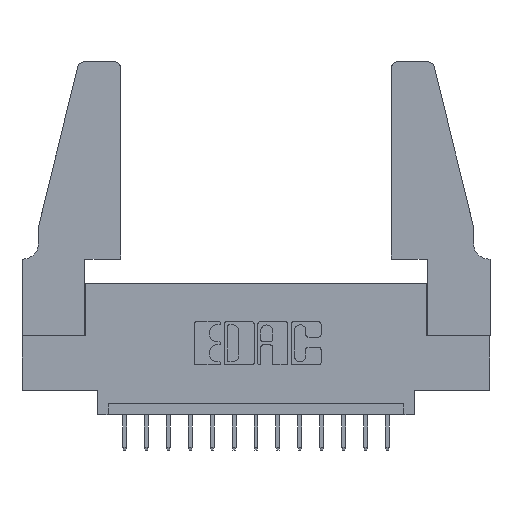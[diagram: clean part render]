
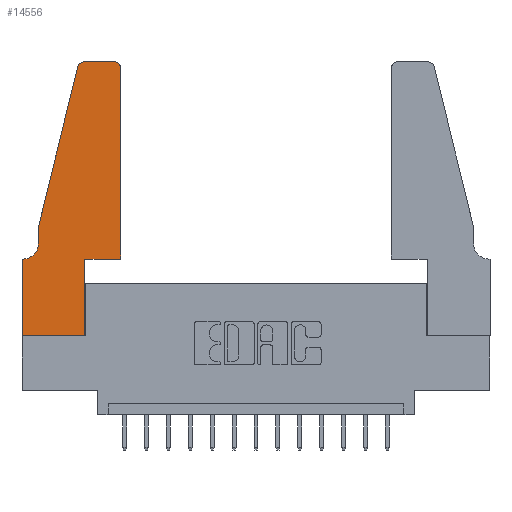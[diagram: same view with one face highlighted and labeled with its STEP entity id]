
A CAD part, top view. The second image highlights one B-rep face of the part: STEP entity #14556.
In plain terms, the highlighted planar face has unit normal (0, 0, 1).
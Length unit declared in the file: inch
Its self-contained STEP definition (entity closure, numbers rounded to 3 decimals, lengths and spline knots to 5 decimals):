
#431 = VERTEX_POINT ( 'NONE', #9113 ) ;
#618 = ORIENTED_EDGE ( 'NONE', *, *, #7225, .T. ) ;
#1413 = VERTEX_POINT ( 'NONE', #5186 ) ;
#1504 = DIRECTION ( 'NONE',  ( 1., 0., 0. ) ) ;
#1596 = ORIENTED_EDGE ( 'NONE', *, *, #14584, .T. ) ;
#2253 = VECTOR ( 'NONE', #13732, 39.37008 ) ;
#2263 = LINE ( 'NONE', #14678, #5330 ) ;
#2307 = VECTOR ( 'NONE', #3714, 39.37008 ) ;
#2390 = ORIENTED_EDGE ( 'NONE', *, *, #8745, .T. ) ;
#2548 = DIRECTION ( 'NONE',  ( 0., 0., -1. ) ) ;
#2800 = CARTESIAN_POINT ( 'NONE',  ( 0.0755, 0.5, 0.37 ) ) ;
#2885 = VERTEX_POINT ( 'NONE', #3122 ) ;
#3049 = EDGE_CURVE ( 'NONE', #12411, #12459, #2263, .T. ) ;
#3122 = CARTESIAN_POINT ( 'NONE',  ( 0.0755, 0.42, 0.37 ) ) ;
#3233 = ORIENTED_EDGE ( 'NONE', *, *, #5597, .T. ) ;
#3341 = FACE_OUTER_BOUND ( 'NONE', #7376, .T. ) ;
#3390 = ORIENTED_EDGE ( 'NONE', *, *, #9537, .T. ) ;
#3483 = DIRECTION ( 'NONE',  ( -0.239, -0.971, 0. ) ) ;
#3714 = DIRECTION ( 'NONE',  ( 0., -1., 0. ) ) ;
#3907 = CARTESIAN_POINT ( 'NONE',  ( 0.0055, 0.42, 0.37 ) ) ;
#4108 = LINE ( 'NONE', #8143, #4893 ) ;
#4590 = VERTEX_POINT ( 'NONE', #15237 ) ;
#4607 = VERTEX_POINT ( 'NONE', #7533 ) ;
#4775 = CARTESIAN_POINT ( 'NONE',  ( 0.4505, 1.22, 0.37 ) ) ;
#4893 = VECTOR ( 'NONE', #13023, 39.37008 ) ;
#5073 = ORIENTED_EDGE ( 'NONE', *, *, #11135, .T. ) ;
#5146 = VECTOR ( 'NONE', #12433, 39.37008 ) ;
#5186 = CARTESIAN_POINT ( 'NONE',  ( 0.284, 1.25, 0.37 ) ) ;
#5328 = CARTESIAN_POINT ( 'NONE',  ( 0.4205, 1.25, 0.37 ) ) ;
#5330 = VECTOR ( 'NONE', #7192, 39.37008 ) ;
#5489 = EDGE_CURVE ( 'NONE', #8499, #431, #14791, .T. ) ;
#5597 = EDGE_CURVE ( 'NONE', #10582, #7871, #9089, .T. ) ;
#5957 = CIRCLE ( 'NONE', #8160, 0.03 ) ;
#6153 = CARTESIAN_POINT ( 'NONE',  ( 0.284, 1.22, 0.37 ) ) ;
#6260 = DIRECTION ( 'NONE',  ( 0., 0., 1. ) ) ;
#6371 = CARTESIAN_POINT ( 'NONE',  ( 0., 0.35, 0.37 ) ) ;
#6404 = VERTEX_POINT ( 'NONE', #5328 ) ;
#6528 = ORIENTED_EDGE ( 'NONE', *, *, #8474, .T. ) ;
#6616 = PLANE ( 'NONE',  #6833 ) ;
#6763 = DIRECTION ( 'NONE',  ( 0., 1., 0. ) ) ;
#6833 = AXIS2_PLACEMENT_3D ( 'NONE', #10396, #7641, #1504 ) ;
#7036 = VECTOR ( 'NONE', #12118, 39.37008 ) ;
#7192 = DIRECTION ( 'NONE',  ( 0., -1., 0. ) ) ;
#7225 = EDGE_CURVE ( 'NONE', #1413, #4590, #5957, .T. ) ;
#7275 = CIRCLE ( 'NONE', #15596, 0.07 ) ;
#7324 = ORIENTED_EDGE ( 'NONE', *, *, #5489, .T. ) ;
#7376 = EDGE_LOOP ( 'NONE', ( #1596, #618, #9408, #5073, #2390, #11083, #7472, #6528, #7324, #3390, #3233, #7913 ) ) ;
#7472 = ORIENTED_EDGE ( 'NONE', *, *, #3049, .T. ) ;
#7533 = CARTESIAN_POINT ( 'NONE',  ( 0.0055, 0.35, 0.37 ) ) ;
#7641 = DIRECTION ( 'NONE',  ( 0., 0., 1. ) ) ;
#7871 = VERTEX_POINT ( 'NONE', #4775 ) ;
#7913 = ORIENTED_EDGE ( 'NONE', *, *, #10476, .T. ) ;
#8143 = CARTESIAN_POINT ( 'NONE',  ( 0.2605, 1.25, 0.37 ) ) ;
#8160 = AXIS2_PLACEMENT_3D ( 'NONE', #6153, #6260, #13027 ) ;
#8455 = LINE ( 'NONE', #15906, #5146 ) ;
#8474 = EDGE_CURVE ( 'NONE', #12459, #8499, #8455, .T. ) ;
#8494 = DIRECTION ( 'NONE',  ( 1., 0., 0. ) ) ;
#8499 = VERTEX_POINT ( 'NONE', #15851 ) ;
#8745 = EDGE_CURVE ( 'NONE', #2885, #4607, #7275, .T. ) ;
#8752 = DIRECTION ( 'NONE',  ( -1., 0., 0. ) ) ;
#8912 = AXIS2_PLACEMENT_3D ( 'NONE', #14722, #15969, #8494 ) ;
#9089 = LINE ( 'NONE', #9173, #9872 ) ;
#9113 = CARTESIAN_POINT ( 'NONE',  ( 0.2865, 0.35, 0.37 ) ) ;
#9173 = CARTESIAN_POINT ( 'NONE',  ( 0.4505, 0.35, 0.37 ) ) ;
#9408 = ORIENTED_EDGE ( 'NONE', *, *, #11956, .T. ) ;
#9411 = LINE ( 'NONE', #9849, #2307 ) ;
#9445 = CARTESIAN_POINT ( 'NONE',  ( 0.4505, 0.35, 0.37 ) ) ;
#9537 = EDGE_CURVE ( 'NONE', #431, #10582, #12461, .T. ) ;
#9649 = CIRCLE ( 'NONE', #8912, 0.03 ) ;
#9849 = CARTESIAN_POINT ( 'NONE',  ( 0.0755, 0.5, 0.37 ) ) ;
#9872 = VECTOR ( 'NONE', #6763, 39.37008 ) ;
#10396 = CARTESIAN_POINT ( 'NONE',  ( 0., 0.35, 0.37 ) ) ;
#10476 = EDGE_CURVE ( 'NONE', #7871, #6404, #9649, .T. ) ;
#10582 = VERTEX_POINT ( 'NONE', #11516 ) ;
#10778 = VECTOR ( 'NONE', #3483, 39.37008 ) ;
#10928 = CARTESIAN_POINT ( 'NONE',  ( 0.2865, 0.35, 0.37 ) ) ;
#10948 = LINE ( 'NONE', #11166, #2253 ) ;
#11083 = ORIENTED_EDGE ( 'NONE', *, *, #12357, .T. ) ;
#11135 = EDGE_CURVE ( 'NONE', #15074, #2885, #9411, .T. ) ;
#11166 = CARTESIAN_POINT ( 'NONE',  ( 0.0755, 0.35, 0.37 ) ) ;
#11516 = CARTESIAN_POINT ( 'NONE',  ( 0.4505, 0.35, 0.37 ) ) ;
#11871 = CARTESIAN_POINT ( 'NONE',  ( 0.0755, 0.5, 0.37 ) ) ;
#11956 = EDGE_CURVE ( 'NONE', #4590, #15074, #14098, .T. ) ;
#12118 = DIRECTION ( 'NONE',  ( 1., 0., 0. ) ) ;
#12357 = EDGE_CURVE ( 'NONE', #4607, #12411, #10948, .T. ) ;
#12411 = VERTEX_POINT ( 'NONE', #6371 ) ;
#12433 = DIRECTION ( 'NONE',  ( 1., 0., 0. ) ) ;
#12459 = VERTEX_POINT ( 'NONE', #13430 ) ;
#12461 = LINE ( 'NONE', #9445, #7036 ) ;
#13023 = DIRECTION ( 'NONE',  ( -1., 0., 0. ) ) ;
#13027 = DIRECTION ( 'NONE',  ( 1., 0., 0. ) ) ;
#13430 = CARTESIAN_POINT ( 'NONE',  ( 0., 0., 0.37 ) ) ;
#13732 = DIRECTION ( 'NONE',  ( -1., 0., 0. ) ) ;
#14098 = LINE ( 'NONE', #11871, #10778 ) ;
#14556 = ADVANCED_FACE ( 'NONE', ( #3341 ), #6616, .T. ) ;
#14582 = VECTOR ( 'NONE', #14707, 39.37008 ) ;
#14584 = EDGE_CURVE ( 'NONE', #6404, #1413, #4108, .T. ) ;
#14678 = CARTESIAN_POINT ( 'NONE',  ( 0., 0., 0.37 ) ) ;
#14707 = DIRECTION ( 'NONE',  ( 0., 1., 0. ) ) ;
#14722 = CARTESIAN_POINT ( 'NONE',  ( 0.4205, 1.22, 0.37 ) ) ;
#14791 = LINE ( 'NONE', #10928, #14582 ) ;
#15074 = VERTEX_POINT ( 'NONE', #2800 ) ;
#15237 = CARTESIAN_POINT ( 'NONE',  ( 0.25487, 1.22718, 0.37 ) ) ;
#15596 = AXIS2_PLACEMENT_3D ( 'NONE', #3907, #2548, #8752 ) ;
#15851 = CARTESIAN_POINT ( 'NONE',  ( 0.2865, 0., 0.37 ) ) ;
#15906 = CARTESIAN_POINT ( 'NONE',  ( 0., 0., 0.37 ) ) ;
#15969 = DIRECTION ( 'NONE',  ( 0., 0., 1. ) ) ;
